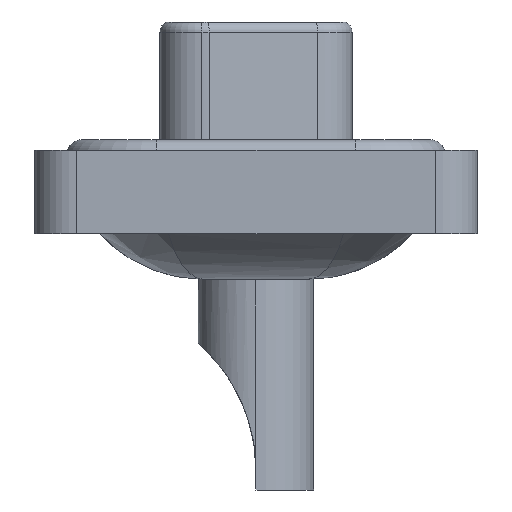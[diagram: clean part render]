
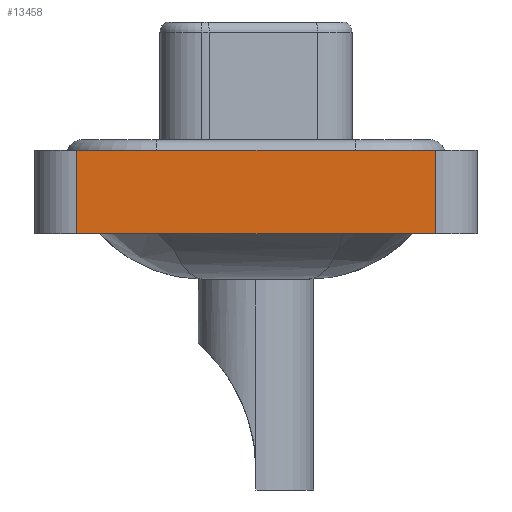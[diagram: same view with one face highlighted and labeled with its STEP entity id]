
A CAD part, left-side view. The second image highlights one B-rep face of the part: STEP entity #13458.
In plain terms, the highlighted planar face has unit normal (-1, 0, 0).
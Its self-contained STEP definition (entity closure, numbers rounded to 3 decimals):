
#444 = LINE ( 'NONE', #10794, #3033 ) ;
#456 = DIRECTION ( 'NONE',  ( 0., 0., 1. ) ) ;
#664 = ORIENTED_EDGE ( 'NONE', *, *, #1933, .F. ) ;
#790 = DIRECTION ( 'NONE',  ( 0., -1., 0. ) ) ;
#892 = CARTESIAN_POINT ( 'NONE',  ( -7.25, 8.55, -3.6 ) ) ;
#1187 = EDGE_CURVE ( 'NONE', #8090, #8367, #9299, .T. ) ;
#1933 = EDGE_CURVE ( 'NONE', #8367, #8360, #13900, .T. ) ;
#2049 = ORIENTED_EDGE ( 'NONE', *, *, #1187, .F. ) ;
#3033 = VECTOR ( 'NONE', #7366, 1000. ) ;
#3090 = VECTOR ( 'NONE', #4772, 1000. ) ;
#3358 = EDGE_CURVE ( 'NONE', #8090, #13767, #444, .T. ) ;
#3943 = EDGE_CURVE ( 'NONE', #13767, #8360, #6934, .T. ) ;
#4471 = DIRECTION ( 'NONE',  ( 0., 0., 1. ) ) ;
#4475 = ORIENTED_EDGE ( 'NONE', *, *, #3358, .T. ) ;
#4772 = DIRECTION ( 'NONE',  ( 0., 0., 1. ) ) ;
#5497 = ORIENTED_EDGE ( 'NONE', *, *, #3943, .T. ) ;
#5719 = VECTOR ( 'NONE', #790, 1000. ) ;
#6231 = DIRECTION ( 'NONE',  ( -1., 0., 0. ) ) ;
#6934 = LINE ( 'NONE', #12660, #8022 ) ;
#7366 = DIRECTION ( 'NONE',  ( 0., -1., 0. ) ) ;
#7376 = CARTESIAN_POINT ( 'NONE',  ( -7.25, -8.55, -3.6 ) ) ;
#8022 = VECTOR ( 'NONE', #4471, 1000. ) ;
#8090 = VERTEX_POINT ( 'NONE', #892 ) ;
#8360 = VERTEX_POINT ( 'NONE', #12060 ) ;
#8367 = VERTEX_POINT ( 'NONE', #13365 ) ;
#9089 = CARTESIAN_POINT ( 'NONE',  ( -7.25, -8.55, 0.4 ) ) ;
#9299 = LINE ( 'NONE', #13953, #3090 ) ;
#10794 = CARTESIAN_POINT ( 'NONE',  ( -7.25, -8.55, -3.6 ) ) ;
#11409 = CARTESIAN_POINT ( 'NONE',  ( -7.25, -8.55, -3.6 ) ) ;
#12060 = CARTESIAN_POINT ( 'NONE',  ( -7.25, -8.55, 0.4 ) ) ;
#12487 = EDGE_LOOP ( 'NONE', ( #5497, #664, #2049, #4475 ) ) ;
#12660 = CARTESIAN_POINT ( 'NONE',  ( -7.25, -8.55, -3.6 ) ) ;
#13027 = PLANE ( 'NONE',  #13030 ) ;
#13030 = AXIS2_PLACEMENT_3D ( 'NONE', #7376, #6231, #456 ) ;
#13365 = CARTESIAN_POINT ( 'NONE',  ( -7.25, 8.55, 0.4 ) ) ;
#13458 = ADVANCED_FACE ( 'NONE', ( #14112 ), #13027, .T. ) ;
#13767 = VERTEX_POINT ( 'NONE', #11409 ) ;
#13900 = LINE ( 'NONE', #9089, #5719 ) ;
#13953 = CARTESIAN_POINT ( 'NONE',  ( -7.25, 8.55, -3.6 ) ) ;
#14112 = FACE_OUTER_BOUND ( 'NONE', #12487, .T. ) ;
